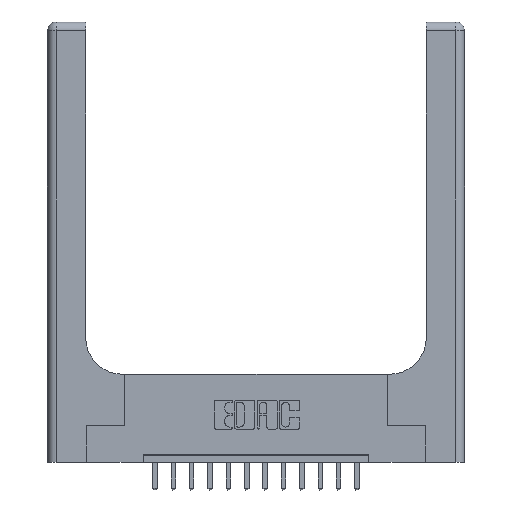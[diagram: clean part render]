
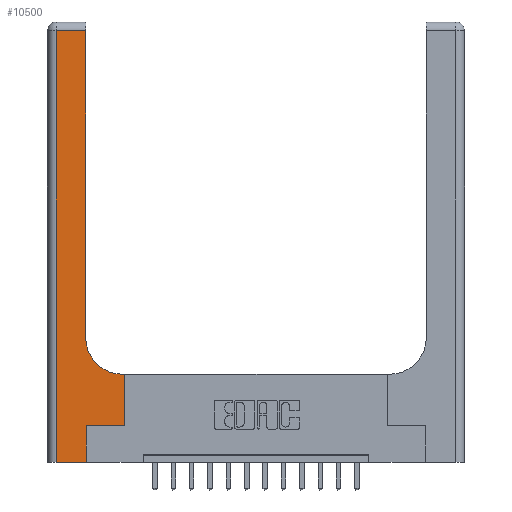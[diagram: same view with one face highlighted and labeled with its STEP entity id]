
A CAD part, top view. The second image highlights one B-rep face of the part: STEP entity #10500.
In plain terms, the highlighted planar face has unit normal (0, 0, 1).
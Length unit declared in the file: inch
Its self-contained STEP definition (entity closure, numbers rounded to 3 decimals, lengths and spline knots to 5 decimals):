
#118 = LINE ( 'NONE', #9588, #13777 ) ;
#120 = AXIS2_PLACEMENT_3D ( 'NONE', #13704, #14905, #5697 ) ;
#640 = ORIENTED_EDGE ( 'NONE', *, *, #13655, .T. ) ;
#1092 = VERTEX_POINT ( 'NONE', #6913 ) ;
#1155 = CIRCLE ( 'NONE', #120, 0.25 ) ;
#1381 = EDGE_CURVE ( 'NONE', #14759, #8804, #14186, .T. ) ;
#1620 = CARTESIAN_POINT ( 'NONE',  ( 0.06, 0., 0.37 ) ) ;
#1903 = VERTEX_POINT ( 'NONE', #6301 ) ;
#2264 = EDGE_CURVE ( 'NONE', #3212, #14759, #118, .T. ) ;
#2641 = CARTESIAN_POINT ( 'NONE',  ( 0., 2.94, 0.37 ) ) ;
#3025 = EDGE_CURVE ( 'NONE', #7166, #3212, #7959, .T. ) ;
#3212 = VERTEX_POINT ( 'NONE', #7294 ) ;
#3706 = DIRECTION ( 'NONE',  ( 0., 1., 0. ) ) ;
#3717 = CARTESIAN_POINT ( 'NONE',  ( 0., 0., 0.37 ) ) ;
#3731 = VECTOR ( 'NONE', #15548, 39.37008 ) ;
#4052 = EDGE_CURVE ( 'NONE', #5115, #7166, #14646, .T. ) ;
#4569 = CARTESIAN_POINT ( 'NONE',  ( 0., 3., 0.37 ) ) ;
#5115 = VERTEX_POINT ( 'NONE', #16601 ) ;
#5291 = CARTESIAN_POINT ( 'NONE',  ( 0.265, 0.25, 0.37 ) ) ;
#5340 = ORIENTED_EDGE ( 'NONE', *, *, #13801, .T. ) ;
#5689 = ORIENTED_EDGE ( 'NONE', *, *, #10068, .T. ) ;
#5697 = DIRECTION ( 'NONE',  ( 1., 0., 0. ) ) ;
#5897 = CARTESIAN_POINT ( 'NONE',  ( 0.265, 0., 0.37 ) ) ;
#6237 = ORIENTED_EDGE ( 'NONE', *, *, #15761, .T. ) ;
#6301 = CARTESIAN_POINT ( 'NONE',  ( 0.51, 0.6, 0.37 ) ) ;
#6326 = VECTOR ( 'NONE', #11639, 39.37008 ) ;
#6465 = ORIENTED_EDGE ( 'NONE', *, *, #9021, .T. ) ;
#6913 = CARTESIAN_POINT ( 'NONE',  ( 0.528, 0.25, 0.37 ) ) ;
#7062 = LINE ( 'NONE', #15937, #8438 ) ;
#7166 = VERTEX_POINT ( 'NONE', #15941 ) ;
#7294 = CARTESIAN_POINT ( 'NONE',  ( 0.06, 2.94, 0.37 ) ) ;
#7452 = VERTEX_POINT ( 'NONE', #5291 ) ;
#7959 = LINE ( 'NONE', #2641, #10386 ) ;
#8045 = EDGE_LOOP ( 'NONE', ( #14045, #10324, #13928, #12876, #6237, #5689, #5340, #6465, #640 ) ) ;
#8438 = VECTOR ( 'NONE', #10692, 39.37008 ) ;
#8444 = DIRECTION ( 'NONE',  ( 0., -1., 0. ) ) ;
#8804 = VERTEX_POINT ( 'NONE', #5897 ) ;
#9007 = LINE ( 'NONE', #12870, #9822 ) ;
#9021 = EDGE_CURVE ( 'NONE', #13366, #1903, #9007, .T. ) ;
#9158 = DIRECTION ( 'NONE',  ( 1., 0., 0. ) ) ;
#9588 = CARTESIAN_POINT ( 'NONE',  ( 0.06, 3., 0.37 ) ) ;
#9772 = LINE ( 'NONE', #11581, #6326 ) ;
#9822 = VECTOR ( 'NONE', #15532, 39.37008 ) ;
#10068 = EDGE_CURVE ( 'NONE', #7452, #1092, #9772, .T. ) ;
#10324 = ORIENTED_EDGE ( 'NONE', *, *, #3025, .T. ) ;
#10386 = VECTOR ( 'NONE', #13037, 39.37008 ) ;
#10500 = ADVANCED_FACE ( 'NONE', ( #12219 ), #12296, .F. ) ;
#10659 = LINE ( 'NONE', #13185, #3731 ) ;
#10692 = DIRECTION ( 'NONE',  ( 0., 1., 0. ) ) ;
#11581 = CARTESIAN_POINT ( 'NONE',  ( 0.265, 0.25, 0.37 ) ) ;
#11639 = DIRECTION ( 'NONE',  ( 1., 0., 0. ) ) ;
#12219 = FACE_OUTER_BOUND ( 'NONE', #8045, .T. ) ;
#12296 = PLANE ( 'NONE',  #13111 ) ;
#12832 = CARTESIAN_POINT ( 'NONE',  ( 0.528, 0.6, 0.37 ) ) ;
#12870 = CARTESIAN_POINT ( 'NONE',  ( 0.26, 0.6, 0.37 ) ) ;
#12876 = ORIENTED_EDGE ( 'NONE', *, *, #1381, .T. ) ;
#13037 = DIRECTION ( 'NONE',  ( -1., 0., 0. ) ) ;
#13111 = AXIS2_PLACEMENT_3D ( 'NONE', #4569, #14706, #15981 ) ;
#13185 = CARTESIAN_POINT ( 'NONE',  ( 0.265, 0., 0.37 ) ) ;
#13366 = VERTEX_POINT ( 'NONE', #12832 ) ;
#13409 = VECTOR ( 'NONE', #9158, 39.37008 ) ;
#13655 = EDGE_CURVE ( 'NONE', #1903, #5115, #1155, .T. ) ;
#13704 = CARTESIAN_POINT ( 'NONE',  ( 0.51, 0.85, 0.37 ) ) ;
#13777 = VECTOR ( 'NONE', #8444, 39.37008 ) ;
#13801 = EDGE_CURVE ( 'NONE', #1092, #13366, #7062, .T. ) ;
#13928 = ORIENTED_EDGE ( 'NONE', *, *, #2264, .T. ) ;
#14045 = ORIENTED_EDGE ( 'NONE', *, *, #4052, .T. ) ;
#14186 = LINE ( 'NONE', #3717, #13409 ) ;
#14646 = LINE ( 'NONE', #16506, #15026 ) ;
#14706 = DIRECTION ( 'NONE',  ( 0., 0., -1. ) ) ;
#14759 = VERTEX_POINT ( 'NONE', #1620 ) ;
#14905 = DIRECTION ( 'NONE',  ( 0., 0., -1. ) ) ;
#15026 = VECTOR ( 'NONE', #3706, 39.37008 ) ;
#15532 = DIRECTION ( 'NONE',  ( -1., 0., 0. ) ) ;
#15548 = DIRECTION ( 'NONE',  ( 0., 1., 0. ) ) ;
#15761 = EDGE_CURVE ( 'NONE', #8804, #7452, #10659, .T. ) ;
#15937 = CARTESIAN_POINT ( 'NONE',  ( 0.528, 0.25, 0.37 ) ) ;
#15941 = CARTESIAN_POINT ( 'NONE',  ( 0.26, 2.94, 0.37 ) ) ;
#15981 = DIRECTION ( 'NONE',  ( -1., 0., 0. ) ) ;
#16506 = CARTESIAN_POINT ( 'NONE',  ( 0.26, 3., 0.37 ) ) ;
#16601 = CARTESIAN_POINT ( 'NONE',  ( 0.26, 0.85, 0.37 ) ) ;
